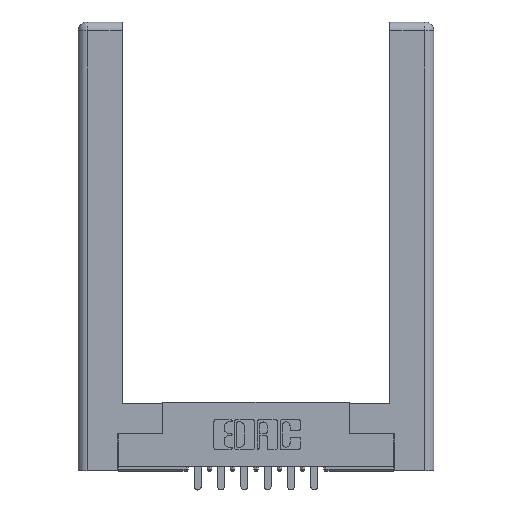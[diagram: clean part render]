
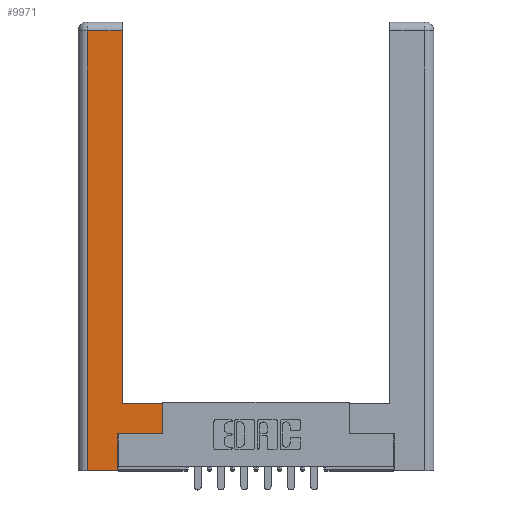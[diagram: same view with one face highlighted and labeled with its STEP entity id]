
A CAD part, top view. The second image highlights one B-rep face of the part: STEP entity #9971.
In plain terms, the highlighted planar face has unit normal (0, 0, 1).
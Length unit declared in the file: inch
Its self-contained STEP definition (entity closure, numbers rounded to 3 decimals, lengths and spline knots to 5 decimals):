
#422 = VERTEX_POINT ( 'NONE', #12004 ) ;
#540 = ORIENTED_EDGE ( 'NONE', *, *, #921, .T. ) ;
#700 = VECTOR ( 'NONE', #2718, 39.37008 ) ;
#738 = LINE ( 'NONE', #1278, #11287 ) ;
#918 = VERTEX_POINT ( 'NONE', #9065 ) ;
#921 = EDGE_CURVE ( 'NONE', #7613, #5219, #12734, .T. ) ;
#969 = ORIENTED_EDGE ( 'NONE', *, *, #12244, .T. ) ;
#1278 = CARTESIAN_POINT ( 'NONE',  ( 0.295, 3., 0. ) ) ;
#1519 = VERTEX_POINT ( 'NONE', #5388 ) ;
#2221 = VECTOR ( 'NONE', #2265, 39.37008 ) ;
#2265 = DIRECTION ( 'NONE',  ( 0., 1., 0. ) ) ;
#2272 = DIRECTION ( 'NONE',  ( -1., 0., 0. ) ) ;
#2295 = AXIS2_PLACEMENT_3D ( 'NONE', #3762, #5853, #4804 ) ;
#2718 = DIRECTION ( 'NONE',  ( 0., 1., 0. ) ) ;
#2775 = DIRECTION ( 'NONE',  ( 1., 0., 0. ) ) ;
#2823 = LINE ( 'NONE', #4554, #12231 ) ;
#3065 = LINE ( 'NONE', #11729, #11040 ) ;
#3120 = EDGE_CURVE ( 'NONE', #918, #6658, #11928, .T. ) ;
#3207 = CARTESIAN_POINT ( 'NONE',  ( 0.295, 0.45, 0. ) ) ;
#3762 = CARTESIAN_POINT ( 'NONE',  ( 0., 0., 0. ) ) ;
#3775 = LINE ( 'NONE', #9749, #700 ) ;
#4357 = DIRECTION ( 'NONE',  ( 0., 1., 0. ) ) ;
#4554 = CARTESIAN_POINT ( 'NONE',  ( 0.295, 0.45, 0. ) ) ;
#4804 = DIRECTION ( 'NONE',  ( -1., 0., 0. ) ) ;
#5219 = VERTEX_POINT ( 'NONE', #6054 ) ;
#5388 = CARTESIAN_POINT ( 'NONE',  ( 0.565, 0.245, 0. ) ) ;
#5513 = DIRECTION ( 'NONE',  ( 0., -1., 0. ) ) ;
#5853 = DIRECTION ( 'NONE',  ( 0., 0., -1. ) ) ;
#6054 = CARTESIAN_POINT ( 'NONE',  ( 0.265, 0., 0. ) ) ;
#6099 = VECTOR ( 'NONE', #2272, 39.37008 ) ;
#6190 = EDGE_CURVE ( 'NONE', #6658, #7613, #3065, .T. ) ;
#6441 = VERTEX_POINT ( 'NONE', #8218 ) ;
#6658 = VERTEX_POINT ( 'NONE', #7231 ) ;
#6943 = VECTOR ( 'NONE', #8570, 39.37008 ) ;
#7001 = ORIENTED_EDGE ( 'NONE', *, *, #13247, .T. ) ;
#7231 = CARTESIAN_POINT ( 'NONE',  ( 0.0615, 2.94, 0. ) ) ;
#7408 = ORIENTED_EDGE ( 'NONE', *, *, #12491, .T. ) ;
#7536 = CARTESIAN_POINT ( 'NONE',  ( 0.565, 0.245, 0. ) ) ;
#7561 = DIRECTION ( 'NONE',  ( -1., 0., 0. ) ) ;
#7613 = VERTEX_POINT ( 'NONE', #9694 ) ;
#7997 = EDGE_LOOP ( 'NONE', ( #969, #11333, #9143, #540, #7001, #12683, #12395, #7408 ) ) ;
#8218 = CARTESIAN_POINT ( 'NONE',  ( 0.565, 0.45, 0. ) ) ;
#8570 = DIRECTION ( 'NONE',  ( 1., 0., 0. ) ) ;
#9065 = CARTESIAN_POINT ( 'NONE',  ( 0.295, 2.94, 0. ) ) ;
#9094 = FACE_OUTER_BOUND ( 'NONE', #7997, .T. ) ;
#9143 = ORIENTED_EDGE ( 'NONE', *, *, #6190, .T. ) ;
#9694 = CARTESIAN_POINT ( 'NONE',  ( 0.0615, 0., 0. ) ) ;
#9703 = CARTESIAN_POINT ( 'NONE',  ( 0.0615, 2.94, 0. ) ) ;
#9749 = CARTESIAN_POINT ( 'NONE',  ( 0.265, 0.245, 0. ) ) ;
#9971 = ADVANCED_FACE ( 'NONE', ( #9094 ), #10049, .F. ) ;
#10023 = CARTESIAN_POINT ( 'NONE',  ( 0.265, 0., 0. ) ) ;
#10049 = PLANE ( 'NONE',  #2295 ) ;
#10530 = CARTESIAN_POINT ( 'NONE',  ( 0.565, 0.45, 0. ) ) ;
#10905 = EDGE_CURVE ( 'NONE', #1519, #6441, #13255, .T. ) ;
#11040 = VECTOR ( 'NONE', #5513, 39.37008 ) ;
#11075 = VERTEX_POINT ( 'NONE', #3207 ) ;
#11287 = VECTOR ( 'NONE', #4357, 39.37008 ) ;
#11332 = EDGE_CURVE ( 'NONE', #422, #1519, #12426, .T. ) ;
#11333 = ORIENTED_EDGE ( 'NONE', *, *, #3120, .T. ) ;
#11729 = CARTESIAN_POINT ( 'NONE',  ( 0.0615, 0., 0. ) ) ;
#11928 = LINE ( 'NONE', #9703, #6099 ) ;
#12004 = CARTESIAN_POINT ( 'NONE',  ( 0.265, 0.245, 0. ) ) ;
#12231 = VECTOR ( 'NONE', #7561, 39.37008 ) ;
#12244 = EDGE_CURVE ( 'NONE', #11075, #918, #738, .T. ) ;
#12395 = ORIENTED_EDGE ( 'NONE', *, *, #10905, .T. ) ;
#12426 = LINE ( 'NONE', #7536, #6943 ) ;
#12491 = EDGE_CURVE ( 'NONE', #6441, #11075, #2823, .T. ) ;
#12683 = ORIENTED_EDGE ( 'NONE', *, *, #11332, .T. ) ;
#12734 = LINE ( 'NONE', #10023, #12911 ) ;
#12911 = VECTOR ( 'NONE', #2775, 39.37008 ) ;
#13247 = EDGE_CURVE ( 'NONE', #5219, #422, #3775, .T. ) ;
#13255 = LINE ( 'NONE', #10530, #2221 ) ;
